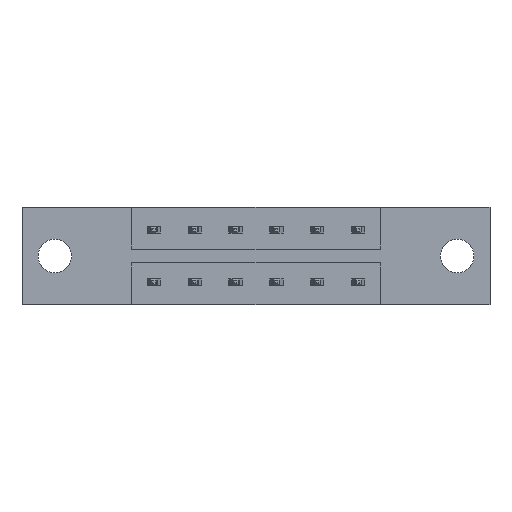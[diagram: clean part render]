
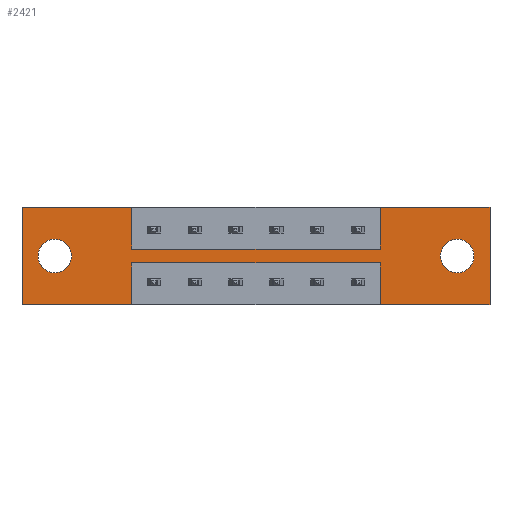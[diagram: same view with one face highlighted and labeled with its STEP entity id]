
A CAD part, front view. The second image highlights one B-rep face of the part: STEP entity #2421.
In plain terms, the highlighted planar face has unit normal (0, -1, 0).
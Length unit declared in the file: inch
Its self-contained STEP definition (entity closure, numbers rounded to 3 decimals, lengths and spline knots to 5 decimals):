
#80 = DIRECTION ( 'NONE',  ( 0., 0., 1. ) ) ;
#88 = CARTESIAN_POINT ( 'NONE',  ( 1.3665, 0., -0.1585 ) ) ;
#121 = CARTESIAN_POINT ( 'NONE',  ( 0.4175, 0., -0.37 ) ) ;
#262 = VERTEX_POINT ( 'NONE', #5257 ) ;
#321 = VERTEX_POINT ( 'NONE', #6829 ) ;
#343 = ORIENTED_EDGE ( 'NONE', *, *, #6068, .F. ) ;
#392 = CARTESIAN_POINT ( 'NONE',  ( 0., 0., -0.37 ) ) ;
#506 = CARTESIAN_POINT ( 'NONE',  ( 1.3665, 0., -0.1585 ) ) ;
#593 = EDGE_CURVE ( 'NONE', #1627, #2948, #4368, .T. ) ;
#612 = DIRECTION ( 'NONE',  ( 0., 0., 1. ) ) ;
#629 = CIRCLE ( 'NONE', #3597, 0.064 ) ;
#675 = DIRECTION ( 'NONE',  ( 0., 1., 0. ) ) ;
#688 = EDGE_CURVE ( 'NONE', #4900, #4943, #5507, .T. ) ;
#707 = CARTESIAN_POINT ( 'NONE',  ( 0.125, 0., -0.185 ) ) ;
#708 = AXIS2_PLACEMENT_3D ( 'NONE', #2056, #6711, #2755 ) ;
#726 = CARTESIAN_POINT ( 'NONE',  ( 1.659, 0., -0.249 ) ) ;
#807 = LINE ( 'NONE', #4339, #7670 ) ;
#860 = VECTOR ( 'NONE', #7993, 39.37008 ) ;
#873 = EDGE_LOOP ( 'NONE', ( #7925, #6482 ) ) ;
#902 = ORIENTED_EDGE ( 'NONE', *, *, #5359, .T. ) ;
#991 = DIRECTION ( 'NONE',  ( 0., 0., -1. ) ) ;
#1044 = CARTESIAN_POINT ( 'NONE',  ( 0.4175, 0., -0.2115 ) ) ;
#1071 = LINE ( 'NONE', #8221, #860 ) ;
#1114 = EDGE_LOOP ( 'NONE', ( #1568, #3664, #343, #5830, #6013, #5728, #7379, #4188, #4389, #1127, #2993, #8113 ) ) ;
#1127 = ORIENTED_EDGE ( 'NONE', *, *, #4434, .F. ) ;
#1128 = VERTEX_POINT ( 'NONE', #2562 ) ;
#1155 = CARTESIAN_POINT ( 'NONE',  ( 1.3665, 0., 0. ) ) ;
#1157 = VERTEX_POINT ( 'NONE', #506 ) ;
#1204 = CARTESIAN_POINT ( 'NONE',  ( 1.784, 0., -0.37 ) ) ;
#1367 = VERTEX_POINT ( 'NONE', #8383 ) ;
#1513 = VECTOR ( 'NONE', #80, 39.37008 ) ;
#1568 = ORIENTED_EDGE ( 'NONE', *, *, #7216, .F. ) ;
#1627 = VERTEX_POINT ( 'NONE', #5855 ) ;
#1641 = PLANE ( 'NONE',  #1733 ) ;
#1708 = VECTOR ( 'NONE', #3505, 39.37008 ) ;
#1709 = CIRCLE ( 'NONE', #4092, 0.064 ) ;
#1733 = AXIS2_PLACEMENT_3D ( 'NONE', #3372, #3642, #7390 ) ;
#1742 = FACE_OUTER_BOUND ( 'NONE', #1114, .T. ) ;
#1794 = CARTESIAN_POINT ( 'NONE',  ( 0.125, 0., -0.185 ) ) ;
#1875 = VECTOR ( 'NONE', #6954, 39.37008 ) ;
#1893 = CARTESIAN_POINT ( 'NONE',  ( 0., 0., -0.37 ) ) ;
#1898 = DIRECTION ( 'NONE',  ( 0., 1., 0. ) ) ;
#2056 = CARTESIAN_POINT ( 'NONE',  ( 1.659, 0., -0.185 ) ) ;
#2419 = DIRECTION ( 'NONE',  ( 0., 0., 1. ) ) ;
#2421 = ADVANCED_FACE ( 'NONE', ( #7066, #3157, #1742 ), #1641, .T. ) ;
#2512 = CIRCLE ( 'NONE', #7051, 0.064 ) ;
#2562 = CARTESIAN_POINT ( 'NONE',  ( 0., 0., 0. ) ) ;
#2755 = DIRECTION ( 'NONE',  ( 0., 0., -1. ) ) ;
#2821 = VECTOR ( 'NONE', #5263, 39.37008 ) ;
#2824 = DIRECTION ( 'NONE',  ( 0., 0., 1. ) ) ;
#2894 = EDGE_CURVE ( 'NONE', #4943, #1157, #1071, .T. ) ;
#2939 = CARTESIAN_POINT ( 'NONE',  ( 0.125, 0., -0.249 ) ) ;
#2948 = VERTEX_POINT ( 'NONE', #121 ) ;
#2980 = VERTEX_POINT ( 'NONE', #726 ) ;
#2993 = ORIENTED_EDGE ( 'NONE', *, *, #593, .F. ) ;
#3097 = CARTESIAN_POINT ( 'NONE',  ( 1.3665, 0., -0.2115 ) ) ;
#3157 = FACE_BOUND ( 'NONE', #873, .T. ) ;
#3347 = VERTEX_POINT ( 'NONE', #4678 ) ;
#3369 = EDGE_CURVE ( 'NONE', #262, #6175, #2512, .T. ) ;
#3372 = CARTESIAN_POINT ( 'NONE',  ( 0., 0., -0.37 ) ) ;
#3504 = LINE ( 'NONE', #392, #8347 ) ;
#3505 = DIRECTION ( 'NONE',  ( 0., 0., -1. ) ) ;
#3597 = AXIS2_PLACEMENT_3D ( 'NONE', #8237, #8230, #8199 ) ;
#3606 = LINE ( 'NONE', #4822, #6846 ) ;
#3612 = EDGE_CURVE ( 'NONE', #3347, #1627, #3606, .T. ) ;
#3642 = DIRECTION ( 'NONE',  ( 0., -1., 0. ) ) ;
#3646 = EDGE_CURVE ( 'NONE', #1157, #5802, #8057, .T. ) ;
#3664 = ORIENTED_EDGE ( 'NONE', *, *, #4123, .F. ) ;
#3975 = VERTEX_POINT ( 'NONE', #1204 ) ;
#3977 = EDGE_CURVE ( 'NONE', #6175, #262, #1709, .T. ) ;
#4092 = AXIS2_PLACEMENT_3D ( 'NONE', #707, #675, #612 ) ;
#4118 = VECTOR ( 'NONE', #7370, 39.37008 ) ;
#4123 = EDGE_CURVE ( 'NONE', #3975, #1367, #7507, .T. ) ;
#4188 = ORIENTED_EDGE ( 'NONE', *, *, #7773, .F. ) ;
#4292 = DIRECTION ( 'NONE',  ( 1., 0., 0. ) ) ;
#4339 = CARTESIAN_POINT ( 'NONE',  ( 0., 0., 0. ) ) ;
#4347 = VERTEX_POINT ( 'NONE', #1893 ) ;
#4368 = LINE ( 'NONE', #1044, #4581 ) ;
#4388 = DIRECTION ( 'NONE',  ( -1., 0., 0. ) ) ;
#4389 = ORIENTED_EDGE ( 'NONE', *, *, #5539, .F. ) ;
#4434 = EDGE_CURVE ( 'NONE', #2948, #4347, #3504, .T. ) ;
#4581 = VECTOR ( 'NONE', #991, 39.37008 ) ;
#4678 = CARTESIAN_POINT ( 'NONE',  ( 1.3665, 0., -0.2115 ) ) ;
#4798 = DIRECTION ( 'NONE',  ( -1., 0., 0. ) ) ;
#4822 = CARTESIAN_POINT ( 'NONE',  ( 0.4175, 0., -0.2115 ) ) ;
#4900 = VERTEX_POINT ( 'NONE', #7028 ) ;
#4943 = VERTEX_POINT ( 'NONE', #6189 ) ;
#5034 = CARTESIAN_POINT ( 'NONE',  ( 0., 0., -0.37 ) ) ;
#5257 = CARTESIAN_POINT ( 'NONE',  ( 0.125, 0., -0.121 ) ) ;
#5263 = DIRECTION ( 'NONE',  ( 0., 0., 1. ) ) ;
#5337 = LINE ( 'NONE', #3097, #6616 ) ;
#5339 = CARTESIAN_POINT ( 'NONE',  ( 0., 0., 0. ) ) ;
#5359 = EDGE_CURVE ( 'NONE', #2980, #6719, #629, .T. ) ;
#5479 = CARTESIAN_POINT ( 'NONE',  ( 1.784, 0., 0. ) ) ;
#5507 = LINE ( 'NONE', #7055, #1875 ) ;
#5539 = EDGE_CURVE ( 'NONE', #4347, #1128, #7420, .T. ) ;
#5557 = LINE ( 'NONE', #5479, #1708 ) ;
#5583 = CARTESIAN_POINT ( 'NONE',  ( 0., 0., 0. ) ) ;
#5728 = ORIENTED_EDGE ( 'NONE', *, *, #2894, .F. ) ;
#5802 = VERTEX_POINT ( 'NONE', #1155 ) ;
#5830 = ORIENTED_EDGE ( 'NONE', *, *, #6961, .F. ) ;
#5855 = CARTESIAN_POINT ( 'NONE',  ( 0.4175, 0., -0.2115 ) ) ;
#6004 = ORIENTED_EDGE ( 'NONE', *, *, #6784, .T. ) ;
#6013 = ORIENTED_EDGE ( 'NONE', *, *, #3646, .F. ) ;
#6068 = EDGE_CURVE ( 'NONE', #321, #3975, #5557, .T. ) ;
#6175 = VERTEX_POINT ( 'NONE', #2939 ) ;
#6189 = CARTESIAN_POINT ( 'NONE',  ( 0.4175, 0., -0.1585 ) ) ;
#6482 = ORIENTED_EDGE ( 'NONE', *, *, #3977, .T. ) ;
#6616 = VECTOR ( 'NONE', #2419, 39.37008 ) ;
#6649 = CARTESIAN_POINT ( 'NONE',  ( 1.659, 0., -0.121 ) ) ;
#6711 = DIRECTION ( 'NONE',  ( 0., 1., 0. ) ) ;
#6719 = VERTEX_POINT ( 'NONE', #6649 ) ;
#6723 = VECTOR ( 'NONE', #4292, 39.37008 ) ;
#6784 = EDGE_CURVE ( 'NONE', #6719, #2980, #7685, .T. ) ;
#6829 = CARTESIAN_POINT ( 'NONE',  ( 1.784, 0., 0. ) ) ;
#6846 = VECTOR ( 'NONE', #4798, 39.37008 ) ;
#6944 = DIRECTION ( 'NONE',  ( 1., 0., 0. ) ) ;
#6954 = DIRECTION ( 'NONE',  ( 0., 0., -1. ) ) ;
#6961 = EDGE_CURVE ( 'NONE', #5802, #321, #8315, .T. ) ;
#7028 = CARTESIAN_POINT ( 'NONE',  ( 0.4175, 0., 0. ) ) ;
#7051 = AXIS2_PLACEMENT_3D ( 'NONE', #1794, #1898, #2824 ) ;
#7055 = CARTESIAN_POINT ( 'NONE',  ( 0.4175, 0., -0.1585 ) ) ;
#7066 = FACE_BOUND ( 'NONE', #7561, .T. ) ;
#7216 = EDGE_CURVE ( 'NONE', #1367, #3347, #5337, .T. ) ;
#7370 = DIRECTION ( 'NONE',  ( -1., 0., 0. ) ) ;
#7379 = ORIENTED_EDGE ( 'NONE', *, *, #688, .F. ) ;
#7390 = DIRECTION ( 'NONE',  ( 0., 0., -1. ) ) ;
#7420 = LINE ( 'NONE', #5339, #2821 ) ;
#7507 = LINE ( 'NONE', #5034, #4118 ) ;
#7561 = EDGE_LOOP ( 'NONE', ( #6004, #902 ) ) ;
#7670 = VECTOR ( 'NONE', #6944, 39.37008 ) ;
#7685 = CIRCLE ( 'NONE', #708, 0.064 ) ;
#7773 = EDGE_CURVE ( 'NONE', #1128, #4900, #807, .T. ) ;
#7925 = ORIENTED_EDGE ( 'NONE', *, *, #3369, .T. ) ;
#7993 = DIRECTION ( 'NONE',  ( 1., 0., 0. ) ) ;
#8057 = LINE ( 'NONE', #88, #1513 ) ;
#8113 = ORIENTED_EDGE ( 'NONE', *, *, #3612, .F. ) ;
#8199 = DIRECTION ( 'NONE',  ( 0., 0., -1. ) ) ;
#8221 = CARTESIAN_POINT ( 'NONE',  ( 0.4175, 0., -0.1585 ) ) ;
#8230 = DIRECTION ( 'NONE',  ( 0., 1., 0. ) ) ;
#8237 = CARTESIAN_POINT ( 'NONE',  ( 1.659, 0., -0.185 ) ) ;
#8315 = LINE ( 'NONE', #5583, #6723 ) ;
#8347 = VECTOR ( 'NONE', #4388, 39.37008 ) ;
#8383 = CARTESIAN_POINT ( 'NONE',  ( 1.3665, 0., -0.37 ) ) ;
